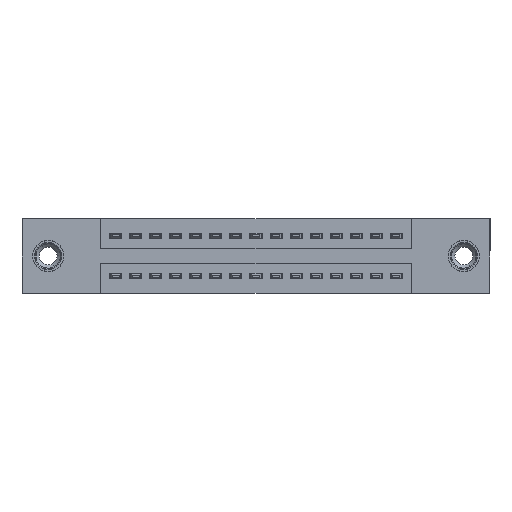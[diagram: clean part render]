
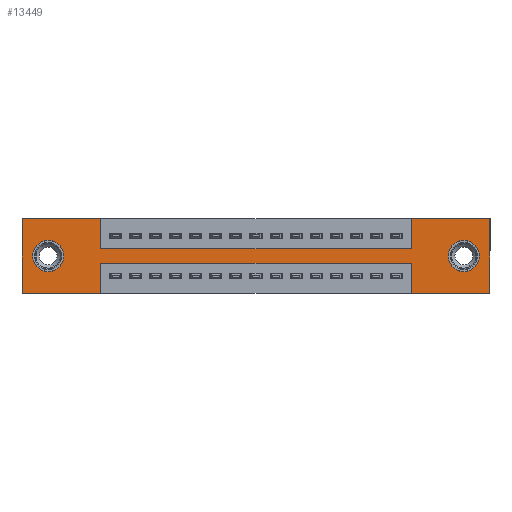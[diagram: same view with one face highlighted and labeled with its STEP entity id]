
A CAD part, front view. The second image highlights one B-rep face of the part: STEP entity #13449.
In plain terms, the highlighted planar face has unit normal (0, -1, 0).
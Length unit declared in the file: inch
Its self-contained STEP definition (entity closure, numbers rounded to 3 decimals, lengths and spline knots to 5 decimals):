
#483 = CARTESIAN_POINT ( 'NONE',  ( 2.205, 0., -0.185 ) ) ;
#662 = ORIENTED_EDGE ( 'NONE', *, *, #10773, .F. ) ;
#720 = LINE ( 'NONE', #18537, #18110 ) ;
#818 = EDGE_CURVE ( 'NONE', #1766, #10622, #15802, .T. ) ;
#830 = DIRECTION ( 'NONE',  ( 0., 0., -1. ) ) ;
#898 = AXIS2_PLACEMENT_3D ( 'NONE', #483, #5094, #17446 ) ;
#1701 = ORIENTED_EDGE ( 'NONE', *, *, #4152, .F. ) ;
#1766 = VERTEX_POINT ( 'NONE', #2100 ) ;
#2100 = CARTESIAN_POINT ( 'NONE',  ( 0.3925, 0., 0. ) ) ;
#2249 = CARTESIAN_POINT ( 'NONE',  ( 2.335, 0., -0.37 ) ) ;
#2257 = ORIENTED_EDGE ( 'NONE', *, *, #17331, .F. ) ;
#2317 = DIRECTION ( 'NONE',  ( 0., 1., 0. ) ) ;
#2408 = VERTEX_POINT ( 'NONE', #13038 ) ;
#2449 = DIRECTION ( 'NONE',  ( 0., 0., 1. ) ) ;
#2816 = ORIENTED_EDGE ( 'NONE', *, *, #6343, .T. ) ;
#3079 = CARTESIAN_POINT ( 'NONE',  ( 1.9425, 0., 0. ) ) ;
#3202 = VERTEX_POINT ( 'NONE', #2249 ) ;
#3229 = CARTESIAN_POINT ( 'NONE',  ( 0.13, 0., -0.263 ) ) ;
#3465 = DIRECTION ( 'NONE',  ( 0., 0., 1. ) ) ;
#3562 = LINE ( 'NONE', #18974, #12011 ) ;
#3697 = ORIENTED_EDGE ( 'NONE', *, *, #9222, .F. ) ;
#4005 = VERTEX_POINT ( 'NONE', #3229 ) ;
#4152 = EDGE_CURVE ( 'NONE', #5550, #2408, #10775, .T. ) ;
#4320 = FACE_BOUND ( 'NONE', #8709, .T. ) ;
#4387 = AXIS2_PLACEMENT_3D ( 'NONE', #9120, #19958, #19894 ) ;
#4400 = ORIENTED_EDGE ( 'NONE', *, *, #6966, .T. ) ;
#4440 = VECTOR ( 'NONE', #14784, 39.37008 ) ;
#4521 = VERTEX_POINT ( 'NONE', #18132 ) ;
#5048 = EDGE_CURVE ( 'NONE', #17940, #7203, #8076, .T. ) ;
#5094 = DIRECTION ( 'NONE',  ( 0., 1., 0. ) ) ;
#5200 = DIRECTION ( 'NONE',  ( 0., -1., 0. ) ) ;
#5416 = CARTESIAN_POINT ( 'NONE',  ( 0.13, 0., -0.185 ) ) ;
#5550 = VERTEX_POINT ( 'NONE', #14340 ) ;
#5563 = ORIENTED_EDGE ( 'NONE', *, *, #13500, .F. ) ;
#5784 = LINE ( 'NONE', #19524, #18088 ) ;
#6005 = VECTOR ( 'NONE', #8650, 39.37008 ) ;
#6169 = DIRECTION ( 'NONE',  ( 0., 0., 1. ) ) ;
#6343 = EDGE_CURVE ( 'NONE', #10370, #12878, #18878, .T. ) ;
#6814 = EDGE_CURVE ( 'NONE', #4005, #4521, #8507, .T. ) ;
#6881 = CARTESIAN_POINT ( 'NONE',  ( 0.3925, 0., -0.37 ) ) ;
#6885 = PLANE ( 'NONE',  #12612 ) ;
#6890 = VECTOR ( 'NONE', #9235, 39.37008 ) ;
#6966 = EDGE_CURVE ( 'NONE', #12878, #10370, #16222, .T. ) ;
#7070 = DIRECTION ( 'NONE',  ( 0., 1., 0. ) ) ;
#7105 = CARTESIAN_POINT ( 'NONE',  ( 0.3925, 0., -0.37 ) ) ;
#7188 = CARTESIAN_POINT ( 'NONE',  ( 0.3925, 0., -0.22 ) ) ;
#7203 = VERTEX_POINT ( 'NONE', #6881 ) ;
#7290 = EDGE_CURVE ( 'NONE', #11763, #17940, #720, .T. ) ;
#7411 = DIRECTION ( 'NONE',  ( 1., 0., 0. ) ) ;
#7658 = EDGE_CURVE ( 'NONE', #12472, #1766, #5784, .T. ) ;
#7902 = ORIENTED_EDGE ( 'NONE', *, *, #5048, .F. ) ;
#8076 = LINE ( 'NONE', #7105, #19642 ) ;
#8507 = CIRCLE ( 'NONE', #17949, 0.078 ) ;
#8513 = CARTESIAN_POINT ( 'NONE',  ( 0.13, 0., -0.185 ) ) ;
#8650 = DIRECTION ( 'NONE',  ( 0., 0., 1. ) ) ;
#8709 = EDGE_LOOP ( 'NONE', ( #19511, #11837 ) ) ;
#9120 = CARTESIAN_POINT ( 'NONE',  ( 2.205, 0., -0.185 ) ) ;
#9222 = EDGE_CURVE ( 'NONE', #19660, #5550, #16593, .T. ) ;
#9235 = DIRECTION ( 'NONE',  ( -1., 0., 0. ) ) ;
#9426 = CARTESIAN_POINT ( 'NONE',  ( 0.3925, 0., 0. ) ) ;
#9548 = ORIENTED_EDGE ( 'NONE', *, *, #7290, .F. ) ;
#9850 = DIRECTION ( 'NONE',  ( 0., 0., -1. ) ) ;
#10089 = CARTESIAN_POINT ( 'NONE',  ( 2.335, 0., 0. ) ) ;
#10107 = EDGE_CURVE ( 'NONE', #2408, #3202, #18701, .T. ) ;
#10116 = EDGE_LOOP ( 'NONE', ( #2816, #4400 ) ) ;
#10370 = VERTEX_POINT ( 'NONE', #18824 ) ;
#10611 = LINE ( 'NONE', #14903, #6005 ) ;
#10622 = VERTEX_POINT ( 'NONE', #19156 ) ;
#10675 = ORIENTED_EDGE ( 'NONE', *, *, #10107, .F. ) ;
#10730 = CARTESIAN_POINT ( 'NONE',  ( 0., 0., -0.37 ) ) ;
#10773 = EDGE_CURVE ( 'NONE', #3202, #14464, #14583, .T. ) ;
#10775 = LINE ( 'NONE', #16774, #18727 ) ;
#11016 = LINE ( 'NONE', #10730, #6890 ) ;
#11178 = ORIENTED_EDGE ( 'NONE', *, *, #818, .F. ) ;
#11483 = ORIENTED_EDGE ( 'NONE', *, *, #19361, .F. ) ;
#11654 = CARTESIAN_POINT ( 'NONE',  ( 0., 0., -0.37 ) ) ;
#11763 = VERTEX_POINT ( 'NONE', #19263 ) ;
#11837 = ORIENTED_EDGE ( 'NONE', *, *, #6814, .T. ) ;
#12011 = VECTOR ( 'NONE', #3465, 39.37008 ) ;
#12472 = VERTEX_POINT ( 'NONE', #16975 ) ;
#12612 = AXIS2_PLACEMENT_3D ( 'NONE', #14437, #5200, #17614 ) ;
#12613 = EDGE_LOOP ( 'NONE', ( #7902, #9548, #16994, #662, #10675, #1701, #3697, #2257, #11178, #14234, #5563, #11483 ) ) ;
#12675 = VERTEX_POINT ( 'NONE', #14196 ) ;
#12768 = DIRECTION ( 'NONE',  ( -1., 0., 0. ) ) ;
#12770 = LINE ( 'NONE', #13677, #15930 ) ;
#12878 = VERTEX_POINT ( 'NONE', #19370 ) ;
#13038 = CARTESIAN_POINT ( 'NONE',  ( 2.335, 0., 0. ) ) ;
#13449 = ADVANCED_FACE ( 'NONE', ( #14473, #4320, #17374 ), #6885, .T. ) ;
#13500 = EDGE_CURVE ( 'NONE', #12675, #12472, #10611, .T. ) ;
#13677 = CARTESIAN_POINT ( 'NONE',  ( 0.3925, 0., -0.15 ) ) ;
#13933 = CARTESIAN_POINT ( 'NONE',  ( 1.9425, 0., -0.37 ) ) ;
#14196 = CARTESIAN_POINT ( 'NONE',  ( 0., 0., -0.37 ) ) ;
#14234 = ORIENTED_EDGE ( 'NONE', *, *, #7658, .F. ) ;
#14340 = CARTESIAN_POINT ( 'NONE',  ( 1.9425, 0., 0. ) ) ;
#14437 = CARTESIAN_POINT ( 'NONE',  ( 0., 0., -0.37 ) ) ;
#14464 = VERTEX_POINT ( 'NONE', #13933 ) ;
#14473 = FACE_BOUND ( 'NONE', #10116, .T. ) ;
#14583 = LINE ( 'NONE', #11654, #4440 ) ;
#14784 = DIRECTION ( 'NONE',  ( -1., 0., 0. ) ) ;
#14903 = CARTESIAN_POINT ( 'NONE',  ( 0., 0., 0. ) ) ;
#15802 = LINE ( 'NONE', #9426, #17475 ) ;
#15930 = VECTOR ( 'NONE', #7411, 39.37008 ) ;
#16075 = VECTOR ( 'NONE', #9850, 39.37008 ) ;
#16222 = CIRCLE ( 'NONE', #898, 0.078 ) ;
#16249 = CARTESIAN_POINT ( 'NONE',  ( 1.9425, 0., -0.15 ) ) ;
#16554 = EDGE_CURVE ( 'NONE', #4521, #4005, #17770, .T. ) ;
#16593 = LINE ( 'NONE', #3079, #19004 ) ;
#16774 = CARTESIAN_POINT ( 'NONE',  ( 0., 0., 0. ) ) ;
#16975 = CARTESIAN_POINT ( 'NONE',  ( 0., 0., 0. ) ) ;
#16982 = DIRECTION ( 'NONE',  ( 0., 0., -1. ) ) ;
#16994 = ORIENTED_EDGE ( 'NONE', *, *, #18363, .F. ) ;
#17331 = EDGE_CURVE ( 'NONE', #10622, #19660, #12770, .T. ) ;
#17374 = FACE_OUTER_BOUND ( 'NONE', #12613, .T. ) ;
#17446 = DIRECTION ( 'NONE',  ( 0., 0., -1. ) ) ;
#17475 = VECTOR ( 'NONE', #16982, 39.37008 ) ;
#17489 = DIRECTION ( 'NONE',  ( 1., 0., 0. ) ) ;
#17614 = DIRECTION ( 'NONE',  ( 0., 0., -1. ) ) ;
#17770 = CIRCLE ( 'NONE', #19874, 0.078 ) ;
#17940 = VERTEX_POINT ( 'NONE', #7188 ) ;
#17949 = AXIS2_PLACEMENT_3D ( 'NONE', #8513, #7070, #19344 ) ;
#18088 = VECTOR ( 'NONE', #18170, 39.37008 ) ;
#18110 = VECTOR ( 'NONE', #12768, 39.37008 ) ;
#18132 = CARTESIAN_POINT ( 'NONE',  ( 0.13, 0., -0.107 ) ) ;
#18170 = DIRECTION ( 'NONE',  ( 1., 0., 0. ) ) ;
#18363 = EDGE_CURVE ( 'NONE', #14464, #11763, #3562, .T. ) ;
#18537 = CARTESIAN_POINT ( 'NONE',  ( 0.3925, 0., -0.22 ) ) ;
#18701 = LINE ( 'NONE', #10089, #16075 ) ;
#18727 = VECTOR ( 'NONE', #17489, 39.37008 ) ;
#18824 = CARTESIAN_POINT ( 'NONE',  ( 2.205, 0., -0.107 ) ) ;
#18878 = CIRCLE ( 'NONE', #4387, 0.078 ) ;
#18974 = CARTESIAN_POINT ( 'NONE',  ( 1.9425, 0., -0.37 ) ) ;
#19004 = VECTOR ( 'NONE', #6169, 39.37008 ) ;
#19156 = CARTESIAN_POINT ( 'NONE',  ( 0.3925, 0., -0.15 ) ) ;
#19263 = CARTESIAN_POINT ( 'NONE',  ( 1.9425, 0., -0.22 ) ) ;
#19344 = DIRECTION ( 'NONE',  ( 0., 0., 1. ) ) ;
#19361 = EDGE_CURVE ( 'NONE', #7203, #12675, #11016, .T. ) ;
#19370 = CARTESIAN_POINT ( 'NONE',  ( 2.205, 0., -0.263 ) ) ;
#19511 = ORIENTED_EDGE ( 'NONE', *, *, #16554, .T. ) ;
#19524 = CARTESIAN_POINT ( 'NONE',  ( 0., 0., 0. ) ) ;
#19642 = VECTOR ( 'NONE', #830, 39.37008 ) ;
#19660 = VERTEX_POINT ( 'NONE', #16249 ) ;
#19874 = AXIS2_PLACEMENT_3D ( 'NONE', #5416, #2317, #2449 ) ;
#19894 = DIRECTION ( 'NONE',  ( 0., 0., -1. ) ) ;
#19958 = DIRECTION ( 'NONE',  ( 0., 1., 0. ) ) ;
